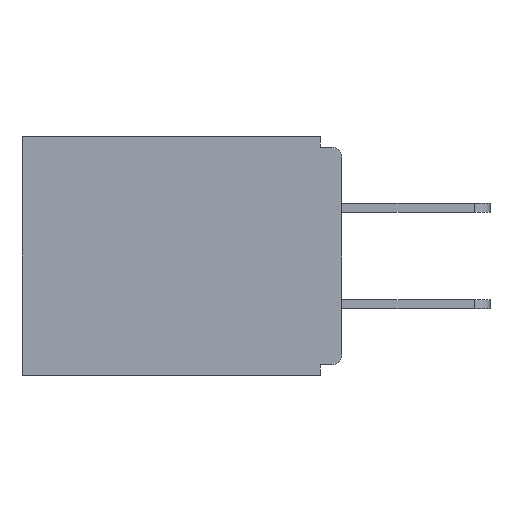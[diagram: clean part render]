
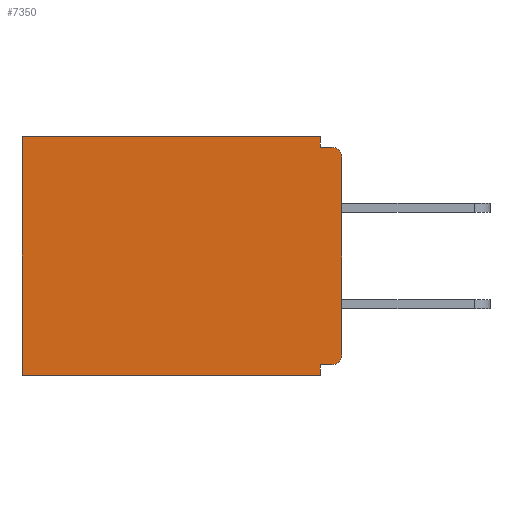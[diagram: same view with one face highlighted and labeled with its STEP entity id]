
A CAD part, left-side view. The second image highlights one B-rep face of the part: STEP entity #7350.
In plain terms, the highlighted planar face has unit normal (-1, 0, 0).
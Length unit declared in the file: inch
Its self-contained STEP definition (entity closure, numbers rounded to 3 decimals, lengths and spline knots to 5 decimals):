
#36 = DIRECTION ( 'NONE',  ( 0., 0., -1. ) ) ;
#540 = DIRECTION ( 'NONE',  ( 0., 0., -1. ) ) ;
#556 = CARTESIAN_POINT ( 'NONE',  ( 0.298, 0., -0.328 ) ) ;
#571 = CARTESIAN_POINT ( 'NONE',  ( 0.298, 0.031, -0.343 ) ) ;
#594 = CARTESIAN_POINT ( 'NONE',  ( 0.298, 0.031, -0.343 ) ) ;
#675 = DIRECTION ( 'NONE',  ( 0., 1., 0. ) ) ;
#707 = DIRECTION ( 'NONE',  ( 0., -1., 0. ) ) ;
#722 = DIRECTION ( 'NONE',  ( 0., 0., -1. ) ) ;
#1046 = CARTESIAN_POINT ( 'NONE',  ( 0.298, 0.015, -0.03 ) ) ;
#1163 = CARTESIAN_POINT ( 'NONE',  ( 0.298, 0.031, -0.328 ) ) ;
#1212 = CARTESIAN_POINT ( 'NONE',  ( 0.298, 0.015, -0.328 ) ) ;
#1417 = DIRECTION ( 'NONE',  ( 0., 1., 0. ) ) ;
#1662 = VECTOR ( 'NONE', #2930, 39.37008 ) ;
#1695 = VERTEX_POINT ( 'NONE', #1163 ) ;
#1721 = VERTEX_POINT ( 'NONE', #7606 ) ;
#2077 = FACE_OUTER_BOUND ( 'NONE', #5797, .T. ) ;
#2292 = ORIENTED_EDGE ( 'NONE', *, *, #5348, .T. ) ;
#2481 = CIRCLE ( 'NONE', #8165, 0.015 ) ;
#2514 = VECTOR ( 'NONE', #9420, 39.37008 ) ;
#2516 = CARTESIAN_POINT ( 'NONE',  ( 0.298, 0.46, -0.343 ) ) ;
#2790 = CIRCLE ( 'NONE', #9870, 0.015 ) ;
#2930 = DIRECTION ( 'NONE',  ( 0., 1., 0. ) ) ;
#2959 = CARTESIAN_POINT ( 'NONE',  ( 0.298, 0.46, 0. ) ) ;
#2963 = VERTEX_POINT ( 'NONE', #5756 ) ;
#3099 = CARTESIAN_POINT ( 'NONE',  ( 0.298, 0., -0.015 ) ) ;
#3118 = VERTEX_POINT ( 'NONE', #6829 ) ;
#3183 = DIRECTION ( 'NONE',  ( -1., 0., 0. ) ) ;
#3367 = VECTOR ( 'NONE', #675, 39.37008 ) ;
#3654 = LINE ( 'NONE', #3099, #8478 ) ;
#3665 = PLANE ( 'NONE',  #9594 ) ;
#3723 = EDGE_CURVE ( 'NONE', #8516, #8834, #7201, .T. ) ;
#3790 = EDGE_CURVE ( 'NONE', #1721, #7978, #6181, .T. ) ;
#3809 = LINE ( 'NONE', #556, #1662 ) ;
#3879 = EDGE_CURVE ( 'NONE', #7978, #3118, #3654, .T. ) ;
#3964 = ORIENTED_EDGE ( 'NONE', *, *, #9047, .F. ) ;
#4121 = LINE ( 'NONE', #7895, #3367 ) ;
#4258 = EDGE_CURVE ( 'NONE', #2963, #9048, #9237, .T. ) ;
#4527 = VECTOR ( 'NONE', #8071, 39.37008 ) ;
#4622 = DIRECTION ( 'NONE',  ( 0., 0., -1. ) ) ;
#4631 = VERTEX_POINT ( 'NONE', #2959 ) ;
#4697 = CARTESIAN_POINT ( 'NONE',  ( 0.298, 0.031, -0.015 ) ) ;
#4797 = EDGE_CURVE ( 'NONE', #4631, #8834, #7439, .T. ) ;
#4849 = CARTESIAN_POINT ( 'NONE',  ( 0.298, 0., 0. ) ) ;
#5003 = DIRECTION ( 'NONE',  ( -1., 0., 0. ) ) ;
#5122 = EDGE_CURVE ( 'NONE', #1721, #4631, #4121, .T. ) ;
#5182 = VECTOR ( 'NONE', #1417, 39.37008 ) ;
#5348 = EDGE_CURVE ( 'NONE', #2963, #3118, #2481, .T. ) ;
#5362 = CARTESIAN_POINT ( 'NONE',  ( 0.298, 0.031, -0.343 ) ) ;
#5529 = ORIENTED_EDGE ( 'NONE', *, *, #9152, .T. ) ;
#5572 = CARTESIAN_POINT ( 'NONE',  ( 0.298, 0.46, 0. ) ) ;
#5734 = ORIENTED_EDGE ( 'NONE', *, *, #4258, .F. ) ;
#5756 = CARTESIAN_POINT ( 'NONE',  ( 0.298, 0., -0.03 ) ) ;
#5797 = EDGE_LOOP ( 'NONE', ( #2292, #10445, #8011, #10354, #6051, #8920, #6910, #3964, #5529, #5734 ) ) ;
#6051 = ORIENTED_EDGE ( 'NONE', *, *, #4797, .T. ) ;
#6135 = DIRECTION ( 'NONE',  ( 1., 0., 0. ) ) ;
#6181 = LINE ( 'NONE', #571, #2514 ) ;
#6239 = CARTESIAN_POINT ( 'NONE',  ( 0.298, 0., -0.343 ) ) ;
#6368 = CARTESIAN_POINT ( 'NONE',  ( 0.298, 0.015, -0.313 ) ) ;
#6483 = EDGE_CURVE ( 'NONE', #1695, #8516, #10349, .T. ) ;
#6793 = VERTEX_POINT ( 'NONE', #1212 ) ;
#6810 = VECTOR ( 'NONE', #36, 39.37008 ) ;
#6829 = CARTESIAN_POINT ( 'NONE',  ( 0.298, 0.015, -0.015 ) ) ;
#6910 = ORIENTED_EDGE ( 'NONE', *, *, #6483, .F. ) ;
#7201 = LINE ( 'NONE', #6239, #5182 ) ;
#7350 = ADVANCED_FACE ( 'NONE', ( #2077 ), #3665, .F. ) ;
#7439 = LINE ( 'NONE', #5572, #4527 ) ;
#7606 = CARTESIAN_POINT ( 'NONE',  ( 0.298, 0.031, 0. ) ) ;
#7895 = CARTESIAN_POINT ( 'NONE',  ( 0.298, 0., 0. ) ) ;
#7978 = VERTEX_POINT ( 'NONE', #4697 ) ;
#8011 = ORIENTED_EDGE ( 'NONE', *, *, #3790, .F. ) ;
#8071 = DIRECTION ( 'NONE',  ( 0., 0., -1. ) ) ;
#8165 = AXIS2_PLACEMENT_3D ( 'NONE', #1046, #5003, #9024 ) ;
#8478 = VECTOR ( 'NONE', #707, 39.37008 ) ;
#8516 = VERTEX_POINT ( 'NONE', #594 ) ;
#8834 = VERTEX_POINT ( 'NONE', #2516 ) ;
#8920 = ORIENTED_EDGE ( 'NONE', *, *, #3723, .F. ) ;
#9024 = DIRECTION ( 'NONE',  ( 0., 0., -1. ) ) ;
#9047 = EDGE_CURVE ( 'NONE', #6793, #1695, #3809, .T. ) ;
#9048 = VERTEX_POINT ( 'NONE', #9438 ) ;
#9152 = EDGE_CURVE ( 'NONE', #6793, #9048, #2790, .T. ) ;
#9237 = LINE ( 'NONE', #4849, #6810 ) ;
#9275 = CARTESIAN_POINT ( 'NONE',  ( 0.298, 0., 0. ) ) ;
#9420 = DIRECTION ( 'NONE',  ( 0., 0., -1. ) ) ;
#9438 = CARTESIAN_POINT ( 'NONE',  ( 0.298, 0., -0.313 ) ) ;
#9594 = AXIS2_PLACEMENT_3D ( 'NONE', #9275, #6135, #4622 ) ;
#9870 = AXIS2_PLACEMENT_3D ( 'NONE', #6368, #3183, #722 ) ;
#10215 = VECTOR ( 'NONE', #540, 39.37008 ) ;
#10349 = LINE ( 'NONE', #5362, #10215 ) ;
#10354 = ORIENTED_EDGE ( 'NONE', *, *, #5122, .T. ) ;
#10445 = ORIENTED_EDGE ( 'NONE', *, *, #3879, .F. ) ;
